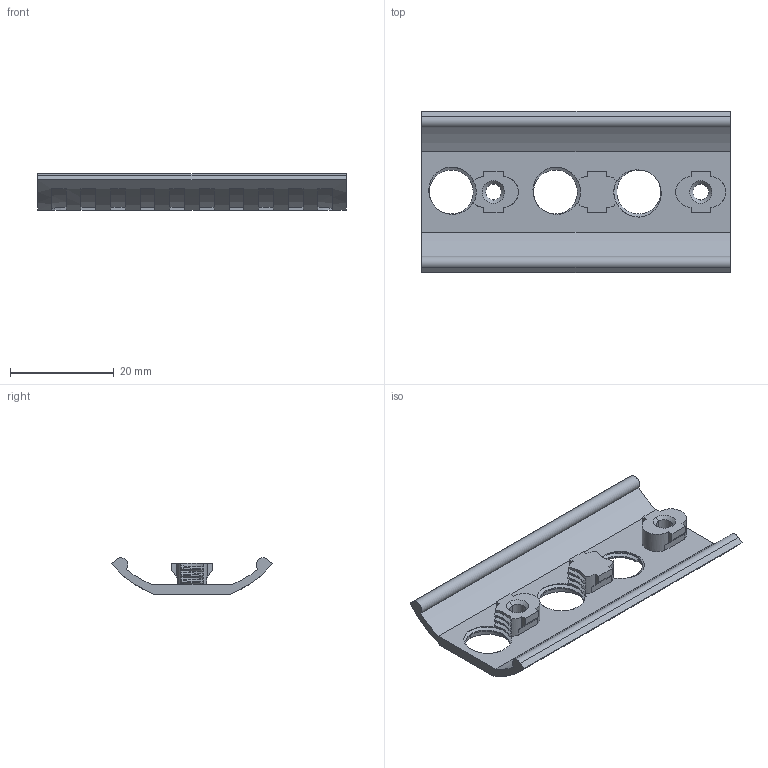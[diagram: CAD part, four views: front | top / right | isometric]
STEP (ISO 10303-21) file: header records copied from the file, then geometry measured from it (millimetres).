
FILE_DESCRIPTION (( 'STEP AP203' ), '1' );
FILE_NAME ('AF-WF-TC-PRT-001-STEP.STEP', '2020-07-22T00:10:30', ( '' ), ( '' ), 'SwSTEP 2.0', 'SolidWorks 2018', '' );
FILE_SCHEMA (( 'CONFIG_CONTROL_DESIGN' ));
Length unit declared in the file: inch
Products named in the file (1): AF-WF-TC-PRT-001-STEP
Bounding box: 59.54 x 31.13 x 7.02 mm (x, y, z)
Volume: 3330.6 mm3; surface area: 5095.9 mm2
Topology: 1 solids, 1 shells, 272 faces, 760 edges, 491 vertices
Faces by surface type: plane 141, cylinder 91, bspline 33, cone 7
Entity records: 13203 total; most frequent: CARTESIAN_POINT 6560, ORIENTED_EDGE 1520, DIRECTION 1245, EDGE_CURVE 760, VERTEX_POINT 491, VECTOR 421, LINE 421, AXIS2_PLACEMENT_3D 412
